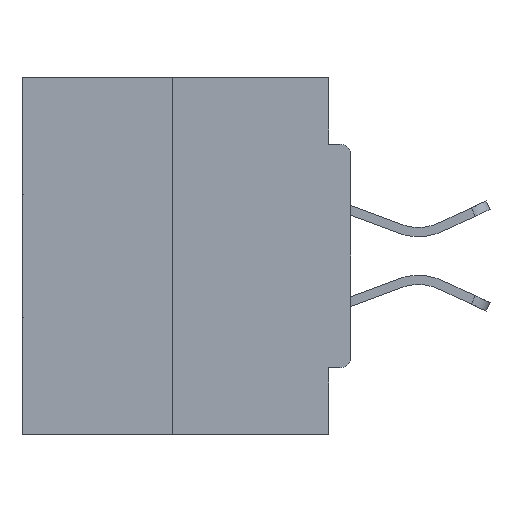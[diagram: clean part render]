
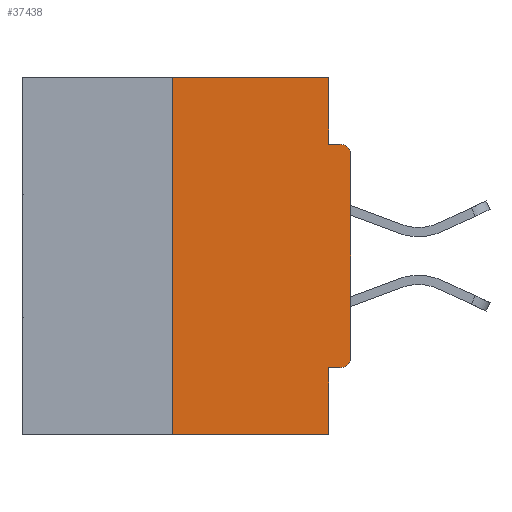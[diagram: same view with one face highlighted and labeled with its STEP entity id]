
A CAD part, left-side view. The second image highlights one B-rep face of the part: STEP entity #37438.
In plain terms, the highlighted planar face has unit normal (-1, 0, 0).
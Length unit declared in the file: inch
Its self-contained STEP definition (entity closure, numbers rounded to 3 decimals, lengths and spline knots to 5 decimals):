
#261 = DIRECTION ( 'NONE',  ( 0., 0., -1. ) ) ;
#712 = DIRECTION ( 'NONE',  ( -1., 0., 0. ) ) ;
#1374 = CARTESIAN_POINT ( 'NONE',  ( 0., 0.46, -0.5 ) ) ;
#1504 = CARTESIAN_POINT ( 'NONE',  ( 0., 0.25, 0. ) ) ;
#1943 = VERTEX_POINT ( 'NONE', #28734 ) ;
#2293 = LINE ( 'NONE', #1374, #9381 ) ;
#2790 = LINE ( 'NONE', #26703, #30201 ) ;
#2930 = VECTOR ( 'NONE', #7428, 39.37008 ) ;
#3102 = ORIENTED_EDGE ( 'NONE', *, *, #22549, .F. ) ;
#4004 = ORIENTED_EDGE ( 'NONE', *, *, #38573, .T. ) ;
#4230 = CARTESIAN_POINT ( 'NONE',  ( 0., 0., -0.4065 ) ) ;
#5212 = AXIS2_PLACEMENT_3D ( 'NONE', #19834, #12873, #25395 ) ;
#6030 = VECTOR ( 'NONE', #36356, 39.37008 ) ;
#6034 = LINE ( 'NONE', #39343, #6030 ) ;
#7106 = DIRECTION ( 'NONE',  ( 0., 0., -1. ) ) ;
#7428 = DIRECTION ( 'NONE',  ( 0., 0., 1. ) ) ;
#7546 = CARTESIAN_POINT ( 'NONE',  ( 0., 0.25, -0.5 ) ) ;
#7889 = DIRECTION ( 'NONE',  ( 0., 0., 1. ) ) ;
#8062 = CARTESIAN_POINT ( 'NONE',  ( 0., 0.031, -0.4065 ) ) ;
#8110 = EDGE_CURVE ( 'NONE', #29432, #8961, #2790, .T. ) ;
#8947 = CARTESIAN_POINT ( 'NONE',  ( 0., 0.031, 0. ) ) ;
#8961 = VERTEX_POINT ( 'NONE', #14511 ) ;
#9381 = VECTOR ( 'NONE', #19522, 39.37008 ) ;
#9398 = VERTEX_POINT ( 'NONE', #39391 ) ;
#9656 = EDGE_CURVE ( 'NONE', #21943, #26603, #10409, .T. ) ;
#10144 = VECTOR ( 'NONE', #261, 39.37008 ) ;
#10409 = LINE ( 'NONE', #18434, #2930 ) ;
#10417 = LINE ( 'NONE', #4230, #27337 ) ;
#11103 = DIRECTION ( 'NONE',  ( 0., -1., 0. ) ) ;
#11704 = EDGE_CURVE ( 'NONE', #8961, #1943, #13911, .T. ) ;
#12855 = CIRCLE ( 'NONE', #35125, 0.015 ) ;
#12873 = DIRECTION ( 'NONE',  ( 1., 0., 0. ) ) ;
#13911 = LINE ( 'NONE', #26054, #22164 ) ;
#14511 = CARTESIAN_POINT ( 'NONE',  ( 0., 0.031, -0.0935 ) ) ;
#15234 = CARTESIAN_POINT ( 'NONE',  ( 0., 0.031, -0.5 ) ) ;
#15287 = CARTESIAN_POINT ( 'NONE',  ( 0., 0.015, -0.3915 ) ) ;
#15428 = LINE ( 'NONE', #15234, #10144 ) ;
#15863 = FACE_OUTER_BOUND ( 'NONE', #23142, .T. ) ;
#17974 = CARTESIAN_POINT ( 'NONE',  ( 0., 0., -0.1085 ) ) ;
#18434 = CARTESIAN_POINT ( 'NONE',  ( 0., 0., 0. ) ) ;
#18613 = EDGE_CURVE ( 'NONE', #27351, #23777, #2293, .T. ) ;
#18943 = VERTEX_POINT ( 'NONE', #29387 ) ;
#19038 = PLANE ( 'NONE',  #5212 ) ;
#19437 = CARTESIAN_POINT ( 'NONE',  ( 0., 0.015, -0.1085 ) ) ;
#19522 = DIRECTION ( 'NONE',  ( 0., -1., 0. ) ) ;
#19834 = CARTESIAN_POINT ( 'NONE',  ( 0., 0.46, 0. ) ) ;
#20934 = DIRECTION ( 'NONE',  ( 0., 0., -1. ) ) ;
#21200 = EDGE_CURVE ( 'NONE', #18943, #29432, #6034, .T. ) ;
#21943 = VERTEX_POINT ( 'NONE', #28705 ) ;
#22164 = VECTOR ( 'NONE', #11103, 39.37008 ) ;
#22454 = EDGE_CURVE ( 'NONE', #38804, #23777, #15428, .T. ) ;
#22549 = EDGE_CURVE ( 'NONE', #9398, #38804, #10417, .T. ) ;
#23142 = EDGE_LOOP ( 'NONE', ( #24591, #37677, #29237, #27081, #3102, #4004, #32952, #25681, #36959, #33871 ) ) ;
#23570 = VECTOR ( 'NONE', #7889, 39.37008 ) ;
#23777 = VERTEX_POINT ( 'NONE', #32807 ) ;
#24591 = ORIENTED_EDGE ( 'NONE', *, *, #21200, .F. ) ;
#25151 = DIRECTION ( 'NONE',  ( 0., 1., 0. ) ) ;
#25395 = DIRECTION ( 'NONE',  ( 0., 0., -1. ) ) ;
#25681 = ORIENTED_EDGE ( 'NONE', *, *, #38686, .T. ) ;
#25993 = DIRECTION ( 'NONE',  ( -1., 0., 0. ) ) ;
#26054 = CARTESIAN_POINT ( 'NONE',  ( 0., 0., -0.0935 ) ) ;
#26603 = VERTEX_POINT ( 'NONE', #17974 ) ;
#26703 = CARTESIAN_POINT ( 'NONE',  ( 0., 0.031, 0. ) ) ;
#27081 = ORIENTED_EDGE ( 'NONE', *, *, #22454, .F. ) ;
#27337 = VECTOR ( 'NONE', #25151, 39.37008 ) ;
#27351 = VERTEX_POINT ( 'NONE', #7546 ) ;
#27472 = AXIS2_PLACEMENT_3D ( 'NONE', #15287, #712, #33211 ) ;
#28705 = CARTESIAN_POINT ( 'NONE',  ( 0., 0., -0.3915 ) ) ;
#28734 = CARTESIAN_POINT ( 'NONE',  ( 0., 0.015, -0.0935 ) ) ;
#28828 = LINE ( 'NONE', #1504, #23570 ) ;
#29237 = ORIENTED_EDGE ( 'NONE', *, *, #18613, .T. ) ;
#29387 = CARTESIAN_POINT ( 'NONE',  ( 0., 0.25, 0. ) ) ;
#29432 = VERTEX_POINT ( 'NONE', #8947 ) ;
#30029 = CIRCLE ( 'NONE', #27472, 0.015 ) ;
#30201 = VECTOR ( 'NONE', #20934, 39.37008 ) ;
#32807 = CARTESIAN_POINT ( 'NONE',  ( 0., 0.031, -0.5 ) ) ;
#32952 = ORIENTED_EDGE ( 'NONE', *, *, #9656, .T. ) ;
#33211 = DIRECTION ( 'NONE',  ( 0., 0., -1. ) ) ;
#33871 = ORIENTED_EDGE ( 'NONE', *, *, #8110, .F. ) ;
#35125 = AXIS2_PLACEMENT_3D ( 'NONE', #19437, #25993, #7106 ) ;
#35927 = EDGE_CURVE ( 'NONE', #27351, #18943, #28828, .T. ) ;
#36356 = DIRECTION ( 'NONE',  ( 0., -1., 0. ) ) ;
#36959 = ORIENTED_EDGE ( 'NONE', *, *, #11704, .F. ) ;
#37438 = ADVANCED_FACE ( 'NONE', ( #15863 ), #19038, .F. ) ;
#37677 = ORIENTED_EDGE ( 'NONE', *, *, #35927, .F. ) ;
#38573 = EDGE_CURVE ( 'NONE', #9398, #21943, #30029, .T. ) ;
#38686 = EDGE_CURVE ( 'NONE', #26603, #1943, #12855, .T. ) ;
#38804 = VERTEX_POINT ( 'NONE', #8062 ) ;
#39343 = CARTESIAN_POINT ( 'NONE',  ( 0., 0.46, 0. ) ) ;
#39391 = CARTESIAN_POINT ( 'NONE',  ( 0., 0.015, -0.4065 ) ) ;
